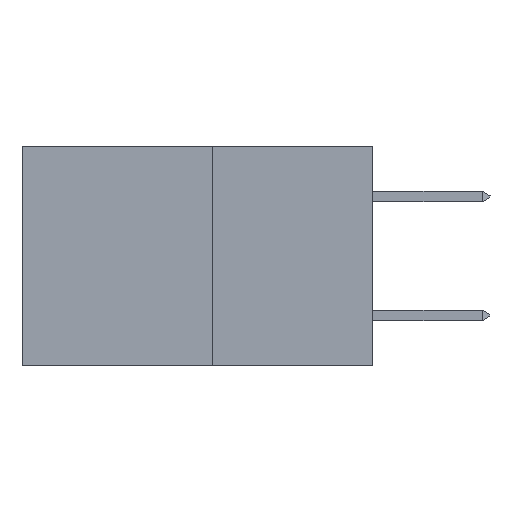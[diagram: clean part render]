
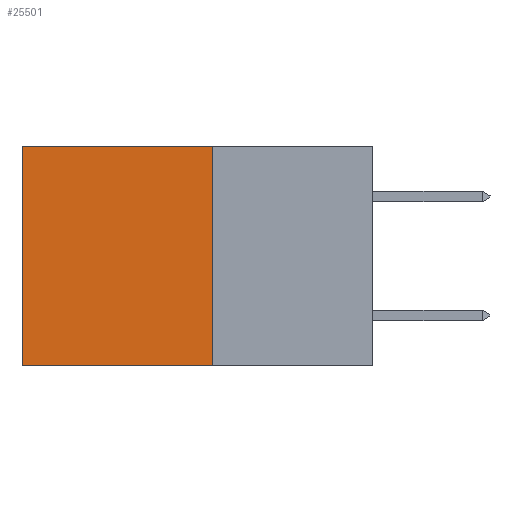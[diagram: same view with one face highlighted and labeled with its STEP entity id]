
A CAD part, left-side view. The second image highlights one B-rep face of the part: STEP entity #25501.
In plain terms, the highlighted planar face has unit normal (-1, 0, 0).
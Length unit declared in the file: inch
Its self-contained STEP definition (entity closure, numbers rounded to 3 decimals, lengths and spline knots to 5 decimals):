
#531 = CARTESIAN_POINT ( 'NONE',  ( 0.277, 0.59, -0.37 ) ) ;
#853 = CARTESIAN_POINT ( 'NONE',  ( 0.277, 0.27, -0.37 ) ) ;
#2374 = ORIENTED_EDGE ( 'NONE', *, *, #26963, .T. ) ;
#2546 = VECTOR ( 'NONE', #15410, 39.37008 ) ;
#2611 = DIRECTION ( 'NONE',  ( 0., 0., -1. ) ) ;
#2701 = EDGE_LOOP ( 'NONE', ( #4620, #3940, #2950, #2374 ) ) ;
#2950 = ORIENTED_EDGE ( 'NONE', *, *, #14805, .F. ) ;
#3940 = ORIENTED_EDGE ( 'NONE', *, *, #24974, .F. ) ;
#4042 = CARTESIAN_POINT ( 'NONE',  ( 0.277, 0.59, -0.37 ) ) ;
#4620 = ORIENTED_EDGE ( 'NONE', *, *, #10014, .T. ) ;
#6476 = VECTOR ( 'NONE', #26900, 39.37008 ) ;
#8211 = VECTOR ( 'NONE', #22000, 39.37008 ) ;
#8996 = PLANE ( 'NONE',  #23092 ) ;
#9603 = VERTEX_POINT ( 'NONE', #531 ) ;
#10014 = EDGE_CURVE ( 'NONE', #17118, #9603, #17443, .T. ) ;
#10076 = VERTEX_POINT ( 'NONE', #18717 ) ;
#11074 = CARTESIAN_POINT ( 'NONE',  ( 0.277, 0.27, -0.37 ) ) ;
#12630 = VECTOR ( 'NONE', #2611, 39.37008 ) ;
#13165 = DIRECTION ( 'NONE',  ( 0., 0., -1. ) ) ;
#14805 = EDGE_CURVE ( 'NONE', #10076, #16449, #18079, .T. ) ;
#14983 = CARTESIAN_POINT ( 'NONE',  ( 0.277, 0.27, -0.37 ) ) ;
#15410 = DIRECTION ( 'NONE',  ( 0., 1., 0. ) ) ;
#16449 = VERTEX_POINT ( 'NONE', #25529 ) ;
#16483 = FACE_OUTER_BOUND ( 'NONE', #2701, .T. ) ;
#17118 = VERTEX_POINT ( 'NONE', #23313 ) ;
#17443 = LINE ( 'NONE', #4042, #6476 ) ;
#18079 = LINE ( 'NONE', #14983, #12630 ) ;
#18565 = LINE ( 'NONE', #19872, #8211 ) ;
#18717 = CARTESIAN_POINT ( 'NONE',  ( 0.277, 0.27, 0. ) ) ;
#19872 = CARTESIAN_POINT ( 'NONE',  ( 0.277, 0.27, 0. ) ) ;
#22000 = DIRECTION ( 'NONE',  ( 0., 1., 0. ) ) ;
#23092 = AXIS2_PLACEMENT_3D ( 'NONE', #11074, #25661, #13165 ) ;
#23313 = CARTESIAN_POINT ( 'NONE',  ( 0.277, 0.59, 0. ) ) ;
#24082 = LINE ( 'NONE', #853, #2546 ) ;
#24974 = EDGE_CURVE ( 'NONE', #16449, #9603, #24082, .T. ) ;
#25501 = ADVANCED_FACE ( 'NONE', ( #16483 ), #8996, .F. ) ;
#25529 = CARTESIAN_POINT ( 'NONE',  ( 0.277, 0.27, -0.37 ) ) ;
#25661 = DIRECTION ( 'NONE',  ( 1., 0., 0. ) ) ;
#26900 = DIRECTION ( 'NONE',  ( 0., 0., -1. ) ) ;
#26963 = EDGE_CURVE ( 'NONE', #10076, #17118, #18565, .T. ) ;
